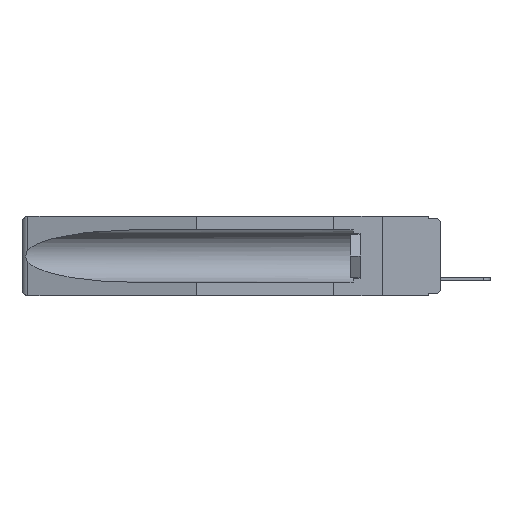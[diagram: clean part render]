
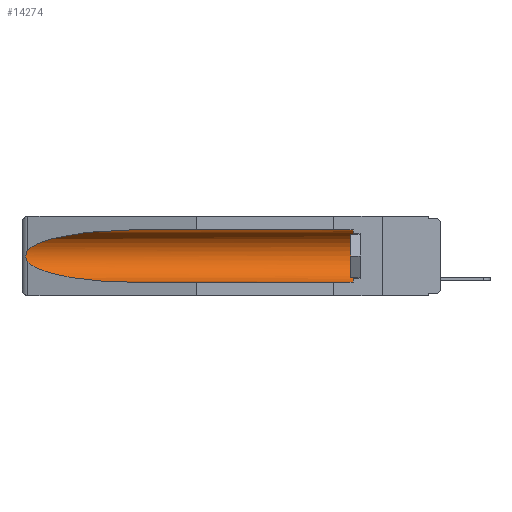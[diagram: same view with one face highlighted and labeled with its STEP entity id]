
A CAD part, left-side view. The second image highlights one B-rep face of the part: STEP entity #14274.
In plain terms, the highlighted cylindrical face has radius 2.857 mm (diameter 5.715 mm), a partial arc.
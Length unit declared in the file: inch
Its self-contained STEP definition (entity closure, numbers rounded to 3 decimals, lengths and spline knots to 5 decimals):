
#675 = CYLINDRICAL_SURFACE ( 'NONE', #22427, 0.1125 ) ;
#830 = CARTESIAN_POINT ( 'NONE',  ( 0.26537, 1.52718, -0.14972 ) ) ;
#1251 = FACE_OUTER_BOUND ( 'NONE', #6372, .T. ) ;
#1374 = CARTESIAN_POINT ( 'NONE',  ( 0.155, -0.30754, -0.284 ) ) ;
#1950 = VERTEX_POINT ( 'NONE', #15753 ) ;
#3258 = CIRCLE ( 'NONE', #17783, 0.1125 ) ;
#3534 = CARTESIAN_POINT ( 'NONE',  ( 0.2675, 1.53308, -0.16763 ) ) ;
#4182 = ORIENTED_EDGE ( 'NONE', *, *, #8396, .T. ) ;
#4468 = CARTESIAN_POINT ( 'NONE',  ( 0.155, 1.07973, -0.059 ) ) ;
#4570 =( BOUNDED_CURVE ( )  B_SPLINE_CURVE ( 3, ( #11587, #15623, #15547, #19203 ),
 .UNSPECIFIED., .F., .F. ) 
 B_SPLINE_CURVE_WITH_KNOTS ( ( 4, 4 ),
 ( 0.1948, 1.5708 ),
 .UNSPECIFIED. ) 
 CURVE ( )  GEOMETRIC_REPRESENTATION_ITEM ( )  RATIONAL_B_SPLINE_CURVE ( ( 1., 0.848, 0.848, 1. ) ) 
 REPRESENTATION_ITEM ( '' )  );
#5302 = CARTESIAN_POINT ( 'NONE',  ( 0.26654, 1.53092, -0.15636 ) ) ;
#5562 = DIRECTION ( 'NONE',  ( 0., 1., 0. ) ) ;
#6320 = ORIENTED_EDGE ( 'NONE', *, *, #12771, .T. ) ;
#6372 = EDGE_LOOP ( 'NONE', ( #13879, #10280, #6395, #17340, #6320, #4182 ) ) ;
#6395 = ORIENTED_EDGE ( 'NONE', *, *, #14631, .T. ) ;
#6484 = EDGE_CURVE ( 'NONE', #18456, #9352, #20962, .T. ) ;
#7347 = DIRECTION ( 'NONE',  ( 0., 0., 1. ) ) ;
#7518 = LINE ( 'NONE', #16741, #8679 ) ;
#8396 = EDGE_CURVE ( 'NONE', #1950, #23238, #7518, .T. ) ;
#8629 = CARTESIAN_POINT ( 'NONE',  ( 0.155, -0.30754, -0.1715 ) ) ;
#8679 = VECTOR ( 'NONE', #5562, 39.37008 ) ;
#9144 = VECTOR ( 'NONE', #13965, 39.37008 ) ;
#9352 = VERTEX_POINT ( 'NONE', #21779 ) ;
#9912 =( BOUNDED_CURVE ( )  B_SPLINE_CURVE ( 3, ( #4468, #19254, #21162, #23008 ),
 .UNSPECIFIED., .F., .F. ) 
 B_SPLINE_CURVE_WITH_KNOTS ( ( 4, 4 ),
 ( 4.71239, 6.08839 ),
 .UNSPECIFIED. ) 
 CURVE ( )  GEOMETRIC_REPRESENTATION_ITEM ( )  RATIONAL_B_SPLINE_CURVE ( ( 1., 0.848, 0.848, 1. ) ) 
 REPRESENTATION_ITEM ( '' )  );
#10280 = ORIENTED_EDGE ( 'NONE', *, *, #21179, .T. ) ;
#11587 = CARTESIAN_POINT ( 'NONE',  ( 0.26537, 1.52718, -0.19328 ) ) ;
#12771 = EDGE_CURVE ( 'NONE', #18456, #1950, #3258, .T. ) ;
#12950 = CARTESIAN_POINT ( 'NONE',  ( 0.155, 0.126, -0.1715 ) ) ;
#13482 = EDGE_CURVE ( 'NONE', #23238, #18212, #9912, .T. ) ;
#13879 = ORIENTED_EDGE ( 'NONE', *, *, #13482, .T. ) ;
#13965 = DIRECTION ( 'NONE',  ( 0., 1., 0. ) ) ;
#14274 = ADVANCED_FACE ( 'NONE', ( #1251 ), #675, .F. ) ;
#14365 = CARTESIAN_POINT ( 'NONE',  ( 0.26537, 1.52718, -0.14972 ) ) ;
#14631 = EDGE_CURVE ( 'NONE', #22885, #9352, #4570, .T. ) ;
#14679 = CARTESIAN_POINT ( 'NONE',  ( 0.26597, 1.5296, -0.19026 ) ) ;
#15258 = CARTESIAN_POINT ( 'NONE',  ( 0.155, 1.07973, -0.059 ) ) ;
#15547 = CARTESIAN_POINT ( 'NONE',  ( 0.21114, 1.30732, -0.284 ) ) ;
#15623 = CARTESIAN_POINT ( 'NONE',  ( 0.25451, 1.48313, -0.24835 ) ) ;
#15753 = CARTESIAN_POINT ( 'NONE',  ( 0.155, 0.126, -0.059 ) ) ;
#16741 = CARTESIAN_POINT ( 'NONE',  ( 0.155, -0.30754, -0.059 ) ) ;
#17340 = ORIENTED_EDGE ( 'NONE', *, *, #6484, .F. ) ;
#17783 = AXIS2_PLACEMENT_3D ( 'NONE', #12950, #21942, #7347 ) ;
#17843 = CARTESIAN_POINT ( 'NONE',  ( 0.26537, 1.52718, -0.19328 ) ) ;
#18124 = CARTESIAN_POINT ( 'NONE',  ( 0.26655, 1.53094, -0.18657 ) ) ;
#18212 = VERTEX_POINT ( 'NONE', #830 ) ;
#18456 = VERTEX_POINT ( 'NONE', #20223 ) ;
#19203 = CARTESIAN_POINT ( 'NONE',  ( 0.155, 1.07973, -0.284 ) ) ;
#19254 = CARTESIAN_POINT ( 'NONE',  ( 0.21114, 1.30732, -0.059 ) ) ;
#19915 = CARTESIAN_POINT ( 'NONE',  ( 0.26537, 1.52718, -0.19328 ) ) ;
#20080 = CARTESIAN_POINT ( 'NONE',  ( 0.2673, 1.5327, -0.16383 ) ) ;
#20223 = CARTESIAN_POINT ( 'NONE',  ( 0.155, 0.126, -0.284 ) ) ;
#20962 = LINE ( 'NONE', #1374, #9144 ) ;
#21162 = CARTESIAN_POINT ( 'NONE',  ( 0.25451, 1.48313, -0.09465 ) ) ;
#21179 = EDGE_CURVE ( 'NONE', #18212, #22885, #21291, .T. ) ;
#21291 = B_SPLINE_CURVE_WITH_KNOTS ( 'NONE', 3,
 ( #14365, #21891, #5302, #20080, #3534, #21662, #23823, #18124, #14679, #19915 ),
 .UNSPECIFIED., .F., .F.,
 ( 4, 2, 2, 2, 4 ),
 ( 0., 0.00029, 0.00058, 0.00087, 0.00117 ),
 .UNSPECIFIED. ) ;
#21662 = CARTESIAN_POINT ( 'NONE',  ( 0.2675, 1.53308, -0.17534 ) ) ;
#21779 = CARTESIAN_POINT ( 'NONE',  ( 0.155, 1.07973, -0.284 ) ) ;
#21891 = CARTESIAN_POINT ( 'NONE',  ( 0.26597, 1.52961, -0.15275 ) ) ;
#21942 = DIRECTION ( 'NONE',  ( 0., -1., 0. ) ) ;
#22427 = AXIS2_PLACEMENT_3D ( 'NONE', #8629, #23373, #23529 ) ;
#22885 = VERTEX_POINT ( 'NONE', #17843 ) ;
#23008 = CARTESIAN_POINT ( 'NONE',  ( 0.26537, 1.52718, -0.14972 ) ) ;
#23238 = VERTEX_POINT ( 'NONE', #15258 ) ;
#23373 = DIRECTION ( 'NONE',  ( 0., 1., 0. ) ) ;
#23529 = DIRECTION ( 'NONE',  ( 0., 0., 1. ) ) ;
#23823 = CARTESIAN_POINT ( 'NONE',  ( 0.2673, 1.53269, -0.17917 ) ) ;
